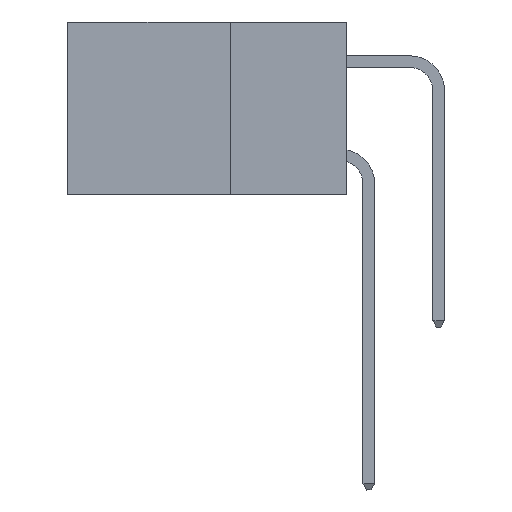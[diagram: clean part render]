
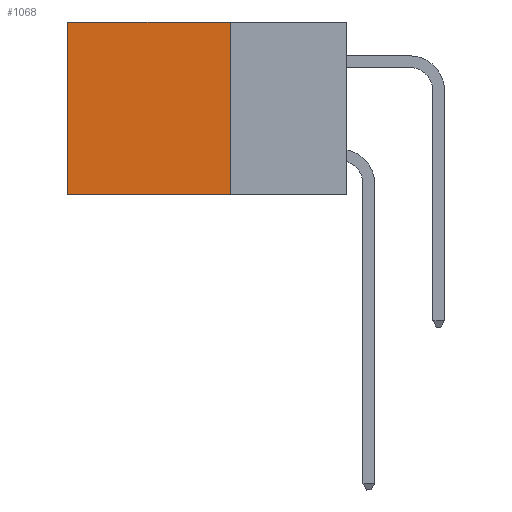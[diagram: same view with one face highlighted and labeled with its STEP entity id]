
A CAD part, left-side view. The second image highlights one B-rep face of the part: STEP entity #1068.
In plain terms, the highlighted planar face has unit normal (-1, 0, 0).
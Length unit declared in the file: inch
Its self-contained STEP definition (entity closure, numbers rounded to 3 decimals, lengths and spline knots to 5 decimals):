
#410 = VECTOR ( 'NONE', #8283, 39.37008 ) ;
#840 = EDGE_LOOP ( 'NONE', ( #28572, #9099, #13936, #8910 ) ) ;
#1068 = ADVANCED_FACE ( 'NONE', ( #11992 ), #10253, .F. ) ;
#1541 = EDGE_CURVE ( 'NONE', #16130, #7147, #17222, .T. ) ;
#2080 = LINE ( 'NONE', #11105, #5915 ) ;
#3209 = CARTESIAN_POINT ( 'NONE',  ( 0.2875, 0.6, 0. ) ) ;
#3557 = DIRECTION ( 'NONE',  ( 0., 0., -1. ) ) ;
#3963 = VECTOR ( 'NONE', #15760, 39.37008 ) ;
#4919 = AXIS2_PLACEMENT_3D ( 'NONE', #21389, #23664, #12796 ) ;
#5278 = CARTESIAN_POINT ( 'NONE',  ( 0.2875, 0.25, 0. ) ) ;
#5915 = VECTOR ( 'NONE', #9120, 39.37008 ) ;
#7147 = VERTEX_POINT ( 'NONE', #26152 ) ;
#8283 = DIRECTION ( 'NONE',  ( 0., 0., -1. ) ) ;
#8910 = ORIENTED_EDGE ( 'NONE', *, *, #15239, .T. ) ;
#9099 = ORIENTED_EDGE ( 'NONE', *, *, #25733, .F. ) ;
#9120 = DIRECTION ( 'NONE',  ( 0., 1., 0. ) ) ;
#9140 = CARTESIAN_POINT ( 'NONE',  ( 0.2875, 0.6, 0. ) ) ;
#10109 = CARTESIAN_POINT ( 'NONE',  ( 0.2875, 0.25, 0. ) ) ;
#10253 = PLANE ( 'NONE',  #4919 ) ;
#10444 = LINE ( 'NONE', #10109, #17447 ) ;
#11105 = CARTESIAN_POINT ( 'NONE',  ( 0.2875, 0.25, -0.37 ) ) ;
#11992 = FACE_OUTER_BOUND ( 'NONE', #840, .T. ) ;
#12796 = DIRECTION ( 'NONE',  ( 0., 0., -1. ) ) ;
#13936 = ORIENTED_EDGE ( 'NONE', *, *, #26018, .F. ) ;
#15239 = EDGE_CURVE ( 'NONE', #18692, #16130, #28126, .T. ) ;
#15760 = DIRECTION ( 'NONE',  ( 0., 1., 0. ) ) ;
#16130 = VERTEX_POINT ( 'NONE', #9140 ) ;
#17222 = LINE ( 'NONE', #3209, #410 ) ;
#17447 = VECTOR ( 'NONE', #3557, 39.37008 ) ;
#18692 = VERTEX_POINT ( 'NONE', #5278 ) ;
#21389 = CARTESIAN_POINT ( 'NONE',  ( 0.2875, 0.25, 0. ) ) ;
#22163 = CARTESIAN_POINT ( 'NONE',  ( 0.2875, 0.25, 0. ) ) ;
#23664 = DIRECTION ( 'NONE',  ( 1., 0., 0. ) ) ;
#25103 = CARTESIAN_POINT ( 'NONE',  ( 0.2875, 0.25, -0.37 ) ) ;
#25242 = VERTEX_POINT ( 'NONE', #25103 ) ;
#25733 = EDGE_CURVE ( 'NONE', #25242, #7147, #2080, .T. ) ;
#26018 = EDGE_CURVE ( 'NONE', #18692, #25242, #10444, .T. ) ;
#26152 = CARTESIAN_POINT ( 'NONE',  ( 0.2875, 0.6, -0.37 ) ) ;
#28126 = LINE ( 'NONE', #22163, #3963 ) ;
#28572 = ORIENTED_EDGE ( 'NONE', *, *, #1541, .T. ) ;
